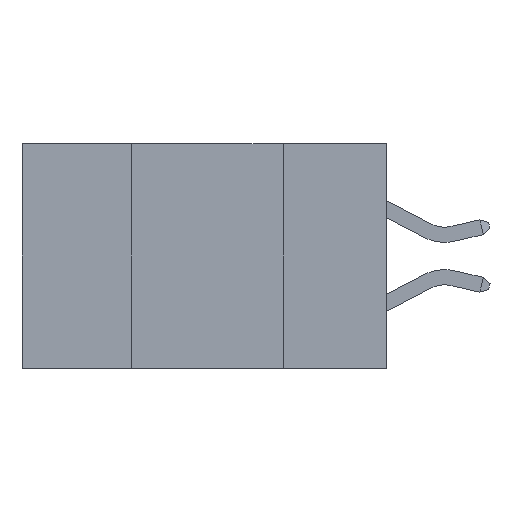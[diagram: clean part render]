
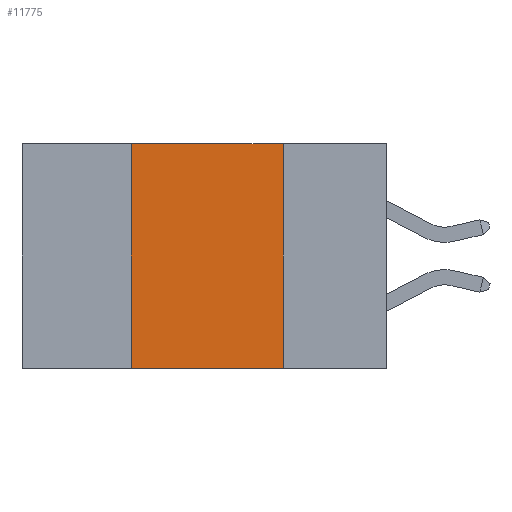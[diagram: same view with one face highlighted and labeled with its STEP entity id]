
A CAD part, left-side view. The second image highlights one B-rep face of the part: STEP entity #11775.
In plain terms, the highlighted planar face has unit normal (-1, 0, 0).
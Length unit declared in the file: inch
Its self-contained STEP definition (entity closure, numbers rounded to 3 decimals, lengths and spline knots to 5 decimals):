
#805 = LINE ( 'NONE', #6235, #7758 ) ;
#1196 = VERTEX_POINT ( 'NONE', #18535 ) ;
#2346 = VERTEX_POINT ( 'NONE', #20295 ) ;
#2638 = ORIENTED_EDGE ( 'NONE', *, *, #24128, .F. ) ;
#3751 = ORIENTED_EDGE ( 'NONE', *, *, #19362, .F. ) ;
#4493 = VERTEX_POINT ( 'NONE', #7899 ) ;
#6235 = CARTESIAN_POINT ( 'NONE',  ( 0., 0.6, 0. ) ) ;
#7208 = PLANE ( 'NONE',  #19631 ) ;
#7758 = VECTOR ( 'NONE', #10517, 39.37008 ) ;
#7786 = DIRECTION ( 'NONE',  ( 0., 0., -1. ) ) ;
#7899 = CARTESIAN_POINT ( 'NONE',  ( 0., 0.17, 0. ) ) ;
#9183 = DIRECTION ( 'NONE',  ( 0., -1., 0. ) ) ;
#9405 = DIRECTION ( 'NONE',  ( 0., 0., -1. ) ) ;
#10291 = VECTOR ( 'NONE', #10380, 39.37008 ) ;
#10380 = DIRECTION ( 'NONE',  ( 0., 0., 1. ) ) ;
#10517 = DIRECTION ( 'NONE',  ( 0., -1., 0. ) ) ;
#11127 = CARTESIAN_POINT ( 'NONE',  ( 0., 0.17, -0.37 ) ) ;
#11775 = ADVANCED_FACE ( 'NONE', ( #19537 ), #7208, .F. ) ;
#12320 = CARTESIAN_POINT ( 'NONE',  ( 0., 0.6, 0. ) ) ;
#14391 = ORIENTED_EDGE ( 'NONE', *, *, #15136, .T. ) ;
#15136 = EDGE_CURVE ( 'NONE', #1196, #25597, #15411, .T. ) ;
#15411 = LINE ( 'NONE', #27996, #30071 ) ;
#16397 = CARTESIAN_POINT ( 'NONE',  ( 0., 0.17, 0. ) ) ;
#16577 = LINE ( 'NONE', #17577, #10291 ) ;
#17577 = CARTESIAN_POINT ( 'NONE',  ( 0., 0.42, 0. ) ) ;
#18535 = CARTESIAN_POINT ( 'NONE',  ( 0., 0.42, -0.37 ) ) ;
#19098 = EDGE_CURVE ( 'NONE', #2346, #4493, #805, .T. ) ;
#19362 = EDGE_CURVE ( 'NONE', #1196, #2346, #16577, .T. ) ;
#19537 = FACE_OUTER_BOUND ( 'NONE', #28430, .T. ) ;
#19631 = AXIS2_PLACEMENT_3D ( 'NONE', #12320, #21824, #7786 ) ;
#20295 = CARTESIAN_POINT ( 'NONE',  ( 0., 0.42, 0. ) ) ;
#21824 = DIRECTION ( 'NONE',  ( 1., 0., 0. ) ) ;
#24042 = VECTOR ( 'NONE', #9405, 39.37008 ) ;
#24128 = EDGE_CURVE ( 'NONE', #4493, #25597, #24777, .T. ) ;
#24777 = LINE ( 'NONE', #16397, #24042 ) ;
#25127 = ORIENTED_EDGE ( 'NONE', *, *, #19098, .F. ) ;
#25597 = VERTEX_POINT ( 'NONE', #11127 ) ;
#27996 = CARTESIAN_POINT ( 'NONE',  ( 0., 0.6, -0.37 ) ) ;
#28430 = EDGE_LOOP ( 'NONE', ( #2638, #25127, #3751, #14391 ) ) ;
#30071 = VECTOR ( 'NONE', #9183, 39.37008 ) ;
